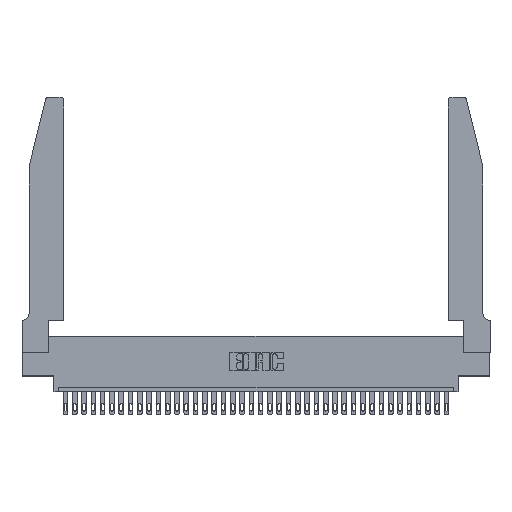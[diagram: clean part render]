
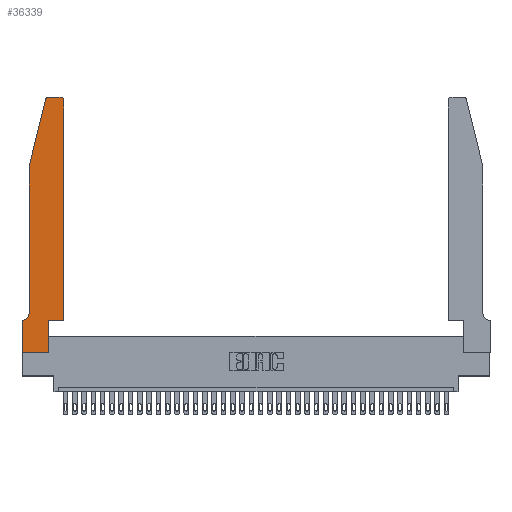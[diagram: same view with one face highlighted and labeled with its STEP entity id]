
A CAD part, top view. The second image highlights one B-rep face of the part: STEP entity #36339.
In plain terms, the highlighted planar face has unit normal (0, 0, 1).
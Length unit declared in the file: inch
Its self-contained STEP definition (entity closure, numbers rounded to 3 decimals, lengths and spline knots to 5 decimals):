
#1023 = AXIS2_PLACEMENT_3D ( 'NONE', #15598, #35390, #35267 ) ;
#1026 = EDGE_CURVE ( 'NONE', #7910, #35178, #24366, .T. ) ;
#1190 = ORIENTED_EDGE ( 'NONE', *, *, #26727, .T. ) ;
#1296 = VECTOR ( 'NONE', #12006, 39.37008 ) ;
#1429 = CARTESIAN_POINT ( 'NONE',  ( 0., 0., 0.37 ) ) ;
#1920 = ORIENTED_EDGE ( 'NONE', *, *, #10307, .T. ) ;
#2717 = DIRECTION ( 'NONE',  ( -1., 0., 0. ) ) ;
#3164 = CARTESIAN_POINT ( 'NONE',  ( 0.4505, 0.35, 0.37 ) ) ;
#3315 = VERTEX_POINT ( 'NONE', #31546 ) ;
#3440 = VERTEX_POINT ( 'NONE', #11786 ) ;
#4324 = CARTESIAN_POINT ( 'NONE',  ( 0.0755, 0.42, 0.37 ) ) ;
#4572 = EDGE_CURVE ( 'NONE', #3440, #9548, #16620, .T. ) ;
#4575 = CIRCLE ( 'NONE', #4873, 0.03 ) ;
#4873 = AXIS2_PLACEMENT_3D ( 'NONE', #11487, #5827, #19596 ) ;
#5746 = CARTESIAN_POINT ( 'NONE',  ( 0.4505, 0.35, 0.37 ) ) ;
#5817 = DIRECTION ( 'NONE',  ( 1., 0., 0. ) ) ;
#5827 = DIRECTION ( 'NONE',  ( 0., 0., 1. ) ) ;
#6152 = ORIENTED_EDGE ( 'NONE', *, *, #16266, .T. ) ;
#6164 = CARTESIAN_POINT ( 'NONE',  ( 0.2605, 2.75, 0.37 ) ) ;
#6754 = DIRECTION ( 'NONE',  ( 0., -1., 0. ) ) ;
#7875 = VECTOR ( 'NONE', #29704, 39.37008 ) ;
#7910 = VERTEX_POINT ( 'NONE', #27158 ) ;
#8193 = LINE ( 'NONE', #24874, #13010 ) ;
#9155 = CARTESIAN_POINT ( 'NONE',  ( 0.2865, 0.35, 0.37 ) ) ;
#9197 = CARTESIAN_POINT ( 'NONE',  ( 0.0755, 2., 0.37 ) ) ;
#9548 = VERTEX_POINT ( 'NONE', #24440 ) ;
#10018 = VERTEX_POINT ( 'NONE', #12709 ) ;
#10088 = CARTESIAN_POINT ( 'NONE',  ( 0., 0., 0.37 ) ) ;
#10307 = EDGE_CURVE ( 'NONE', #10018, #35633, #19328, .T. ) ;
#10366 = VERTEX_POINT ( 'NONE', #21615 ) ;
#10950 = DIRECTION ( 'NONE',  ( 0., 1., 0. ) ) ;
#11487 = CARTESIAN_POINT ( 'NONE',  ( 0.284, 2.72, 0.37 ) ) ;
#11524 = DIRECTION ( 'NONE',  ( 0., 0., -1. ) ) ;
#11786 = CARTESIAN_POINT ( 'NONE',  ( 0., 0., 0.37 ) ) ;
#12006 = DIRECTION ( 'NONE',  ( 0., -1., 0. ) ) ;
#12685 = LINE ( 'NONE', #5746, #34210 ) ;
#12709 = CARTESIAN_POINT ( 'NONE',  ( 0.0755, 2., 0.37 ) ) ;
#12773 = PLANE ( 'NONE',  #1023 ) ;
#13010 = VECTOR ( 'NONE', #2717, 39.37008 ) ;
#13920 = ORIENTED_EDGE ( 'NONE', *, *, #1026, .T. ) ;
#13941 = CARTESIAN_POINT ( 'NONE',  ( 0.4205, 2.72, 0.37 ) ) ;
#15304 = CARTESIAN_POINT ( 'NONE',  ( 0.4205, 2.75, 0.37 ) ) ;
#15452 = EDGE_CURVE ( 'NONE', #23389, #21869, #28036, .T. ) ;
#15598 = CARTESIAN_POINT ( 'NONE',  ( 0., 0.35, 0.37 ) ) ;
#16266 = EDGE_CURVE ( 'NONE', #21869, #7910, #12685, .T. ) ;
#16620 = LINE ( 'NONE', #1429, #7875 ) ;
#17034 = CARTESIAN_POINT ( 'NONE',  ( 0.0055, 0.42, 0.37 ) ) ;
#18122 = EDGE_CURVE ( 'NONE', #26562, #3315, #8193, .T. ) ;
#18173 = ORIENTED_EDGE ( 'NONE', *, *, #18436, .T. ) ;
#18436 = EDGE_CURVE ( 'NONE', #35178, #10366, #26639, .T. ) ;
#19020 = ORIENTED_EDGE ( 'NONE', *, *, #24718, .T. ) ;
#19328 = LINE ( 'NONE', #9197, #1296 ) ;
#19596 = DIRECTION ( 'NONE',  ( 1., 0., 0. ) ) ;
#19626 = ORIENTED_EDGE ( 'NONE', *, *, #15452, .T. ) ;
#19825 = DIRECTION ( 'NONE',  ( 0., 0., 1. ) ) ;
#20222 = ORIENTED_EDGE ( 'NONE', *, *, #26873, .T. ) ;
#21615 = CARTESIAN_POINT ( 'NONE',  ( 0.284, 2.75, 0.37 ) ) ;
#21869 = VERTEX_POINT ( 'NONE', #22048 ) ;
#21914 = LINE ( 'NONE', #10088, #24552 ) ;
#22048 = CARTESIAN_POINT ( 'NONE',  ( 0.4505, 0.35, 0.37 ) ) ;
#22346 = ORIENTED_EDGE ( 'NONE', *, *, #18122, .T. ) ;
#22785 = EDGE_CURVE ( 'NONE', #35633, #26562, #26691, .T. ) ;
#23017 = LINE ( 'NONE', #9155, #31378 ) ;
#23205 = VECTOR ( 'NONE', #28145, 39.37008 ) ;
#23389 = VERTEX_POINT ( 'NONE', #25731 ) ;
#24076 = ORIENTED_EDGE ( 'NONE', *, *, #4572, .T. ) ;
#24366 = CIRCLE ( 'NONE', #30053, 0.03 ) ;
#24440 = CARTESIAN_POINT ( 'NONE',  ( 0.2865, 0., 0.37 ) ) ;
#24552 = VECTOR ( 'NONE', #6754, 39.37008 ) ;
#24718 = EDGE_CURVE ( 'NONE', #3315, #3440, #21914, .T. ) ;
#24874 = CARTESIAN_POINT ( 'NONE',  ( 0.0755, 0.35, 0.37 ) ) ;
#25731 = CARTESIAN_POINT ( 'NONE',  ( 0.2865, 0.35, 0.37 ) ) ;
#25912 = CARTESIAN_POINT ( 'NONE',  ( 0.25487, 2.72718, 0.37 ) ) ;
#25993 = LINE ( 'NONE', #33734, #32595 ) ;
#26562 = VERTEX_POINT ( 'NONE', #29921 ) ;
#26639 = LINE ( 'NONE', #6164, #27062 ) ;
#26691 = CIRCLE ( 'NONE', #34905, 0.07 ) ;
#26727 = EDGE_CURVE ( 'NONE', #10366, #28673, #4575, .T. ) ;
#26873 = EDGE_CURVE ( 'NONE', #9548, #23389, #23017, .T. ) ;
#27062 = VECTOR ( 'NONE', #34552, 39.37008 ) ;
#27158 = CARTESIAN_POINT ( 'NONE',  ( 0.4505, 2.72, 0.37 ) ) ;
#28036 = LINE ( 'NONE', #3164, #23205 ) ;
#28145 = DIRECTION ( 'NONE',  ( 1., 0., 0. ) ) ;
#28184 = DIRECTION ( 'NONE',  ( -0.239, -0.971, 0. ) ) ;
#28673 = VERTEX_POINT ( 'NONE', #25912 ) ;
#28798 = DIRECTION ( 'NONE',  ( 0., 1., 0. ) ) ;
#29319 = FACE_OUTER_BOUND ( 'NONE', #33693, .T. ) ;
#29361 = ORIENTED_EDGE ( 'NONE', *, *, #31440, .T. ) ;
#29704 = DIRECTION ( 'NONE',  ( 1., 0., 0. ) ) ;
#29921 = CARTESIAN_POINT ( 'NONE',  ( 0.0055, 0.35, 0.37 ) ) ;
#30053 = AXIS2_PLACEMENT_3D ( 'NONE', #13941, #19825, #5817 ) ;
#31378 = VECTOR ( 'NONE', #28798, 39.37008 ) ;
#31440 = EDGE_CURVE ( 'NONE', #28673, #10018, #25993, .T. ) ;
#31546 = CARTESIAN_POINT ( 'NONE',  ( 0., 0.35, 0.37 ) ) ;
#32595 = VECTOR ( 'NONE', #28184, 39.37008 ) ;
#33023 = ORIENTED_EDGE ( 'NONE', *, *, #22785, .T. ) ;
#33693 = EDGE_LOOP ( 'NONE', ( #18173, #1190, #29361, #1920, #33023, #22346, #19020, #24076, #20222, #19626, #6152, #13920 ) ) ;
#33734 = CARTESIAN_POINT ( 'NONE',  ( 0.0755, 2., 0.37 ) ) ;
#34132 = DIRECTION ( 'NONE',  ( -1., 0., 0. ) ) ;
#34210 = VECTOR ( 'NONE', #10950, 39.37008 ) ;
#34552 = DIRECTION ( 'NONE',  ( -1., 0., 0. ) ) ;
#34905 = AXIS2_PLACEMENT_3D ( 'NONE', #17034, #11524, #34132 ) ;
#35178 = VERTEX_POINT ( 'NONE', #15304 ) ;
#35267 = DIRECTION ( 'NONE',  ( 1., 0., 0. ) ) ;
#35390 = DIRECTION ( 'NONE',  ( 0., 0., 1. ) ) ;
#35633 = VERTEX_POINT ( 'NONE', #4324 ) ;
#36339 = ADVANCED_FACE ( 'NONE', ( #29319 ), #12773, .T. ) ;
